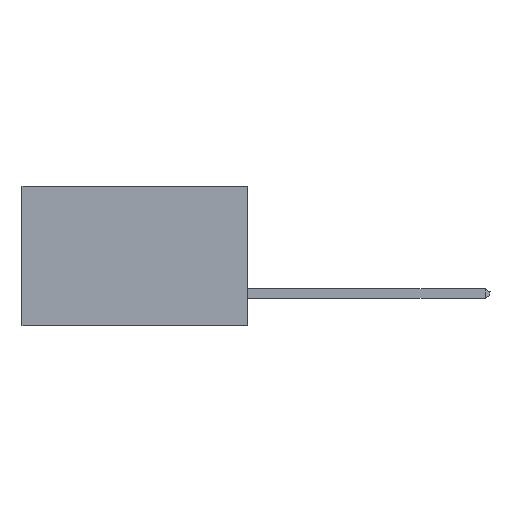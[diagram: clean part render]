
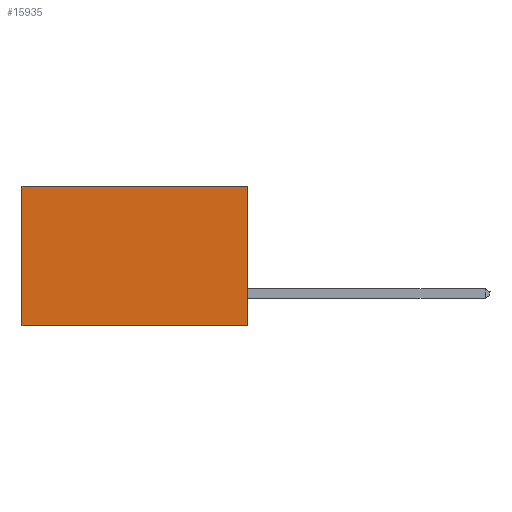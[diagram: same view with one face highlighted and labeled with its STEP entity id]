
A CAD part, left-side view. The second image highlights one B-rep face of the part: STEP entity #15935.
In plain terms, the highlighted planar face has unit normal (-1, 0, 0).
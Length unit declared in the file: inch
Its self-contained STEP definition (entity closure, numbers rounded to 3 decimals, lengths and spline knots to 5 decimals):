
#513 = ORIENTED_EDGE ( 'NONE', *, *, #2919, .T. ) ;
#792 = VECTOR ( 'NONE', #13632, 39.37008 ) ;
#2919 = EDGE_CURVE ( 'NONE', #10171, #19214, #7494, .T. ) ;
#3178 = DIRECTION ( 'NONE',  ( 0., 0., -1. ) ) ;
#3382 = FACE_OUTER_BOUND ( 'NONE', #13051, .T. ) ;
#3790 = AXIS2_PLACEMENT_3D ( 'NONE', #10637, #7061, #16217 ) ;
#7059 = LINE ( 'NONE', #20141, #14338 ) ;
#7061 = DIRECTION ( 'NONE',  ( 1., 0., 0. ) ) ;
#7494 = LINE ( 'NONE', #14754, #18168 ) ;
#8399 = LINE ( 'NONE', #22911, #792 ) ;
#8637 = LINE ( 'NONE', #16249, #19352 ) ;
#8963 = PLANE ( 'NONE',  #3790 ) ;
#9059 = CARTESIAN_POINT ( 'NONE',  ( 0.2615, 0.6, -0.37 ) ) ;
#10171 = VERTEX_POINT ( 'NONE', #20649 ) ;
#10637 = CARTESIAN_POINT ( 'NONE',  ( 0.2615, 0., -0.37 ) ) ;
#11317 = CARTESIAN_POINT ( 'NONE',  ( 0.2615, 0., -0.37 ) ) ;
#13051 = EDGE_LOOP ( 'NONE', ( #14002, #23469, #19665, #513 ) ) ;
#13632 = DIRECTION ( 'NONE',  ( 0., 1., 0. ) ) ;
#13829 = EDGE_CURVE ( 'NONE', #19214, #18914, #7059, .T. ) ;
#14002 = ORIENTED_EDGE ( 'NONE', *, *, #13829, .T. ) ;
#14338 = VECTOR ( 'NONE', #21920, 39.37008 ) ;
#14754 = CARTESIAN_POINT ( 'NONE',  ( 0.2615, 0., 0. ) ) ;
#15403 = EDGE_CURVE ( 'NONE', #10171, #19025, #8637, .T. ) ;
#15935 = ADVANCED_FACE ( 'NONE', ( #3382 ), #8963, .F. ) ;
#16217 = DIRECTION ( 'NONE',  ( 0., 0., -1. ) ) ;
#16249 = CARTESIAN_POINT ( 'NONE',  ( 0.2615, 0., -0.37 ) ) ;
#17103 = EDGE_CURVE ( 'NONE', #19025, #18914, #8399, .T. ) ;
#18168 = VECTOR ( 'NONE', #22009, 39.37008 ) ;
#18914 = VERTEX_POINT ( 'NONE', #9059 ) ;
#19025 = VERTEX_POINT ( 'NONE', #11317 ) ;
#19173 = CARTESIAN_POINT ( 'NONE',  ( 0.2615, 0.6, 0. ) ) ;
#19214 = VERTEX_POINT ( 'NONE', #19173 ) ;
#19352 = VECTOR ( 'NONE', #3178, 39.37008 ) ;
#19665 = ORIENTED_EDGE ( 'NONE', *, *, #15403, .F. ) ;
#20141 = CARTESIAN_POINT ( 'NONE',  ( 0.2615, 0.6, -0.37 ) ) ;
#20649 = CARTESIAN_POINT ( 'NONE',  ( 0.2615, 0., 0. ) ) ;
#21920 = DIRECTION ( 'NONE',  ( 0., 0., -1. ) ) ;
#22009 = DIRECTION ( 'NONE',  ( 0., 1., 0. ) ) ;
#22911 = CARTESIAN_POINT ( 'NONE',  ( 0.2615, 0., -0.37 ) ) ;
#23469 = ORIENTED_EDGE ( 'NONE', *, *, #17103, .F. ) ;
